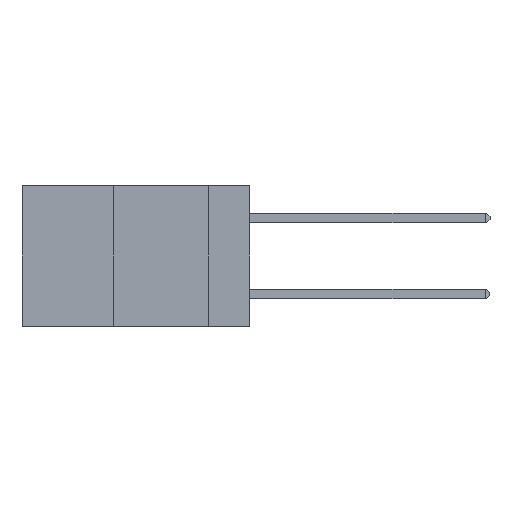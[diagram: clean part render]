
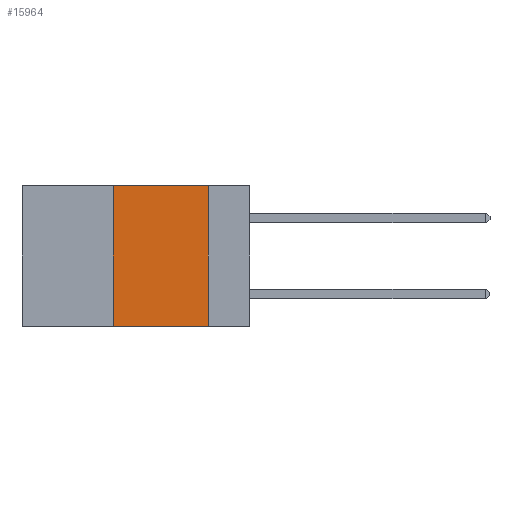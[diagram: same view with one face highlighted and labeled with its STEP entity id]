
A CAD part, left-side view. The second image highlights one B-rep face of the part: STEP entity #15964.
In plain terms, the highlighted planar face has unit normal (-1, 0, 0).
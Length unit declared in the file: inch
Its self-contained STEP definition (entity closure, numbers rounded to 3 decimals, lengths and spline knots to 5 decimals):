
#731 = VECTOR ( 'NONE', #1918, 39.37008 ) ;
#1756 = EDGE_LOOP ( 'NONE', ( #15689, #11505, #15998, #8812 ) ) ;
#1918 = DIRECTION ( 'NONE',  ( 0., -1., 0. ) ) ;
#2440 = PLANE ( 'NONE',  #6443 ) ;
#2630 = CARTESIAN_POINT ( 'NONE',  ( 0., 0.6, -0.37 ) ) ;
#3172 = VERTEX_POINT ( 'NONE', #4905 ) ;
#3522 = VECTOR ( 'NONE', #8817, 39.37008 ) ;
#3589 = EDGE_CURVE ( 'NONE', #3172, #11226, #14587, .T. ) ;
#3690 = DIRECTION ( 'NONE',  ( 0., 0., -1. ) ) ;
#3801 = CARTESIAN_POINT ( 'NONE',  ( 0., 0.11, -0.37 ) ) ;
#4116 = LINE ( 'NONE', #6612, #731 ) ;
#4905 = CARTESIAN_POINT ( 'NONE',  ( 0., 0.11, 0. ) ) ;
#5409 = VECTOR ( 'NONE', #12591, 39.37008 ) ;
#6196 = DIRECTION ( 'NONE',  ( 0., -1., 0. ) ) ;
#6296 = EDGE_CURVE ( 'NONE', #11785, #11226, #11192, .T. ) ;
#6333 = EDGE_CURVE ( 'NONE', #11904, #3172, #4116, .T. ) ;
#6422 = CARTESIAN_POINT ( 'NONE',  ( 0., 0.11, 0. ) ) ;
#6443 = AXIS2_PLACEMENT_3D ( 'NONE', #7428, #11217, #3690 ) ;
#6612 = CARTESIAN_POINT ( 'NONE',  ( 0., 0.6, 0. ) ) ;
#6712 = FACE_OUTER_BOUND ( 'NONE', #1756, .T. ) ;
#7428 = CARTESIAN_POINT ( 'NONE',  ( 0., 0.6, 0. ) ) ;
#7839 = VECTOR ( 'NONE', #6196, 39.37008 ) ;
#8506 = CARTESIAN_POINT ( 'NONE',  ( 0., 0.36, -0.37 ) ) ;
#8812 = ORIENTED_EDGE ( 'NONE', *, *, #6296, .T. ) ;
#8817 = DIRECTION ( 'NONE',  ( 0., 0., 1. ) ) ;
#9481 = EDGE_CURVE ( 'NONE', #11785, #11904, #10571, .T. ) ;
#10571 = LINE ( 'NONE', #16199, #3522 ) ;
#11192 = LINE ( 'NONE', #2630, #7839 ) ;
#11217 = DIRECTION ( 'NONE',  ( 1., 0., 0. ) ) ;
#11226 = VERTEX_POINT ( 'NONE', #3801 ) ;
#11505 = ORIENTED_EDGE ( 'NONE', *, *, #6333, .F. ) ;
#11785 = VERTEX_POINT ( 'NONE', #8506 ) ;
#11904 = VERTEX_POINT ( 'NONE', #16172 ) ;
#12591 = DIRECTION ( 'NONE',  ( 0., 0., -1. ) ) ;
#14587 = LINE ( 'NONE', #6422, #5409 ) ;
#15689 = ORIENTED_EDGE ( 'NONE', *, *, #3589, .F. ) ;
#15964 = ADVANCED_FACE ( 'NONE', ( #6712 ), #2440, .F. ) ;
#15998 = ORIENTED_EDGE ( 'NONE', *, *, #9481, .F. ) ;
#16172 = CARTESIAN_POINT ( 'NONE',  ( 0., 0.36, 0. ) ) ;
#16199 = CARTESIAN_POINT ( 'NONE',  ( 0., 0.36, 0. ) ) ;
